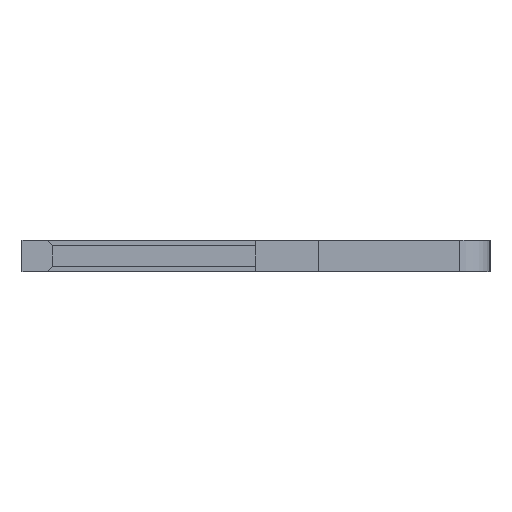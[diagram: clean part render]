
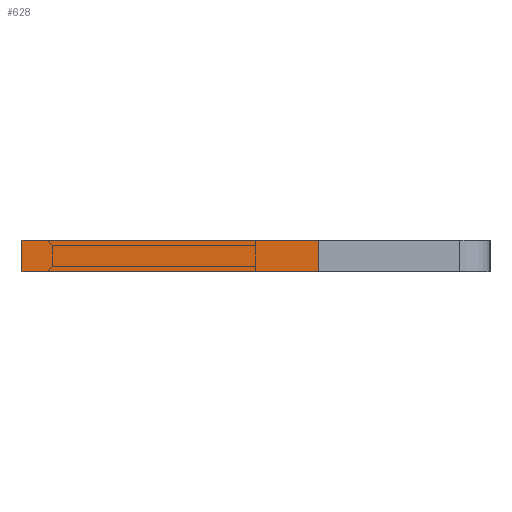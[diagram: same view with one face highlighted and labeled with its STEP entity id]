
A CAD part, left-side view. The second image highlights one B-rep face of the part: STEP entity #628.
In plain terms, the highlighted face is planar.
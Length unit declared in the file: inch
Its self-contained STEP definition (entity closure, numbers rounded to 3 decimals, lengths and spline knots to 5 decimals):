
#79 = VERTEX_POINT ( 'NONE', #931 ) ;
#169 = CARTESIAN_POINT ( 'NONE',  ( 0.01, 0.15, -0.04 ) ) ;
#326 = DIRECTION ( 'NONE',  ( -1., 0., 0. ) ) ;
#554 = ORIENTED_EDGE ( 'NONE', *, *, #1534, .T. ) ;
#628 = ADVANCED_FACE ( 'NONE', ( #1821 ), #1358, .F. ) ;
#648 = DIRECTION ( 'NONE',  ( 0., 0., 1. ) ) ;
#658 = DIRECTION ( 'NONE',  ( 0., 1., 0. ) ) ;
#931 = CARTESIAN_POINT ( 'NONE',  ( -0.01, 0.15, -0.04 ) ) ;
#972 = DIRECTION ( 'NONE',  ( 1., 0., 0. ) ) ;
#1011 = EDGE_CURVE ( 'NONE', #4237, #2064, #4089, .T. ) ;
#1057 = VECTOR ( 'NONE', #658, 39.37008 ) ;
#1355 = DIRECTION ( 'NONE',  ( -1., 0., 0. ) ) ;
#1358 = PLANE ( 'NONE',  #2268 ) ;
#1374 = CARTESIAN_POINT ( 'NONE',  ( 0.01, -0.04, -0.04 ) ) ;
#1479 = ORIENTED_EDGE ( 'NONE', *, *, #3661, .F. ) ;
#1534 = EDGE_CURVE ( 'NONE', #2064, #79, #2246, .T. ) ;
#1821 = FACE_OUTER_BOUND ( 'NONE', #3970, .T. ) ;
#1890 = VECTOR ( 'NONE', #1355, 39.37008 ) ;
#2064 = VERTEX_POINT ( 'NONE', #2124 ) ;
#2124 = CARTESIAN_POINT ( 'NONE',  ( -0.01, -0.04, -0.04 ) ) ;
#2182 = VERTEX_POINT ( 'NONE', #3445 ) ;
#2239 = ORIENTED_EDGE ( 'NONE', *, *, #1011, .T. ) ;
#2246 = LINE ( 'NONE', #4107, #1057 ) ;
#2268 = AXIS2_PLACEMENT_3D ( 'NONE', #3755, #648, #972 ) ;
#2304 = CARTESIAN_POINT ( 'NONE',  ( 0.01, 0.15, -0.04 ) ) ;
#2595 = LINE ( 'NONE', #169, #2803 ) ;
#2803 = VECTOR ( 'NONE', #3869, 39.37008 ) ;
#2902 = LINE ( 'NONE', #2304, #1890 ) ;
#3259 = VECTOR ( 'NONE', #326, 39.37008 ) ;
#3429 = CARTESIAN_POINT ( 'NONE',  ( 0.01, -0.04, -0.04 ) ) ;
#3445 = CARTESIAN_POINT ( 'NONE',  ( 0.01, 0.15, -0.04 ) ) ;
#3582 = ORIENTED_EDGE ( 'NONE', *, *, #3961, .F. ) ;
#3661 = EDGE_CURVE ( 'NONE', #4237, #2182, #2595, .T. ) ;
#3755 = CARTESIAN_POINT ( 'NONE',  ( 0.01, 0.15, -0.04 ) ) ;
#3869 = DIRECTION ( 'NONE',  ( 0., 1., 0. ) ) ;
#3961 = EDGE_CURVE ( 'NONE', #2182, #79, #2902, .T. ) ;
#3970 = EDGE_LOOP ( 'NONE', ( #554, #3582, #1479, #2239 ) ) ;
#4089 = LINE ( 'NONE', #3429, #3259 ) ;
#4107 = CARTESIAN_POINT ( 'NONE',  ( -0.01, 0.15, -0.04 ) ) ;
#4237 = VERTEX_POINT ( 'NONE', #1374 ) ;
